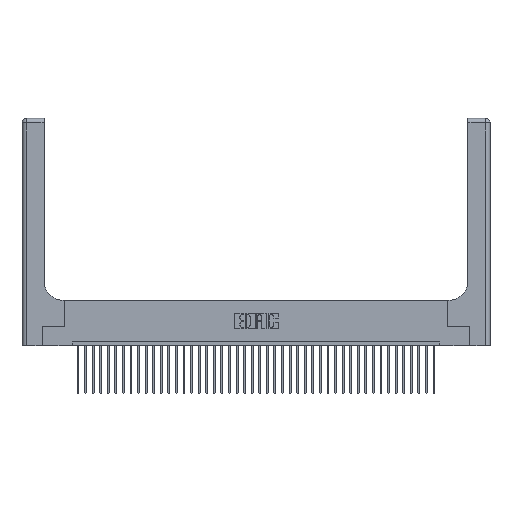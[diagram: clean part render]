
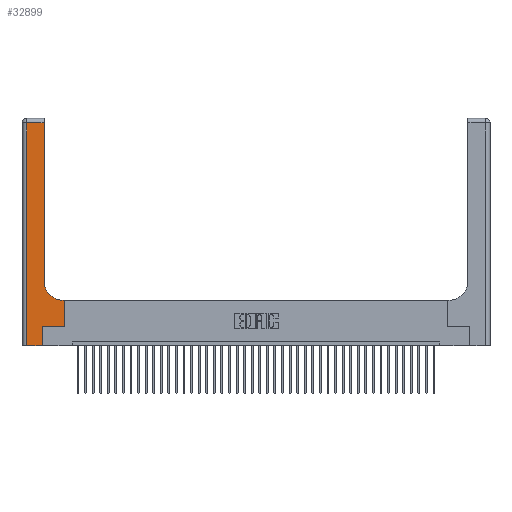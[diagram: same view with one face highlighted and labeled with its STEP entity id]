
A CAD part, top view. The second image highlights one B-rep face of the part: STEP entity #32899.
In plain terms, the highlighted planar face has unit normal (0, 0, 1).
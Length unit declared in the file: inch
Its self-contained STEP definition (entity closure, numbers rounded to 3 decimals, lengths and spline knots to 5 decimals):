
#25 = LINE ( 'NONE', #28274, #21069 ) ;
#470 = ORIENTED_EDGE ( 'NONE', *, *, #32537, .T. ) ;
#648 = CARTESIAN_POINT ( 'NONE',  ( 0., 2.94, 0.37 ) ) ;
#672 = DIRECTION ( 'NONE',  ( 0., 0., -1. ) ) ;
#700 = CARTESIAN_POINT ( 'NONE',  ( 0.269, 0.25, 0.37 ) ) ;
#2259 = CARTESIAN_POINT ( 'NONE',  ( 0.269, 0., 0.37 ) ) ;
#2383 = CARTESIAN_POINT ( 'NONE',  ( 0.5585, 0.6, 0.37 ) ) ;
#2815 = DIRECTION ( 'NONE',  ( 1., 0., 0. ) ) ;
#3543 = DIRECTION ( 'NONE',  ( 0., 1., 0. ) ) ;
#3746 = VERTEX_POINT ( 'NONE', #5873 ) ;
#4926 = LINE ( 'NONE', #5613, #18164 ) ;
#5576 = DIRECTION ( 'NONE',  ( 1., 0., 0. ) ) ;
#5613 = CARTESIAN_POINT ( 'NONE',  ( 0.06, 3., 0.37 ) ) ;
#5708 = VERTEX_POINT ( 'NONE', #24587 ) ;
#5873 = CARTESIAN_POINT ( 'NONE',  ( 0.5415, 0.6, 0.37 ) ) ;
#5874 = CARTESIAN_POINT ( 'NONE',  ( 0.06, 0., 0.37 ) ) ;
#6068 = ORIENTED_EDGE ( 'NONE', *, *, #31612, .T. ) ;
#6712 = CARTESIAN_POINT ( 'NONE',  ( 0., 3., 0.37 ) ) ;
#6886 = VECTOR ( 'NONE', #3543, 39.37008 ) ;
#9248 = LINE ( 'NONE', #35840, #23408 ) ;
#10217 = EDGE_CURVE ( 'NONE', #30166, #11776, #25, .T. ) ;
#10220 = ORIENTED_EDGE ( 'NONE', *, *, #34628, .T. ) ;
#10222 = VECTOR ( 'NONE', #38254, 39.37008 ) ;
#10480 = CARTESIAN_POINT ( 'NONE',  ( 0.06, 2.94, 0.37 ) ) ;
#10695 = EDGE_CURVE ( 'NONE', #19285, #37135, #11729, .T. ) ;
#11729 = LINE ( 'NONE', #14682, #14678 ) ;
#11776 = VERTEX_POINT ( 'NONE', #17389 ) ;
#12494 = ORIENTED_EDGE ( 'NONE', *, *, #20137, .T. ) ;
#12866 = DIRECTION ( 'NONE',  ( -1., 0., 0. ) ) ;
#13947 = DIRECTION ( 'NONE',  ( -1., 0., 0. ) ) ;
#14678 = VECTOR ( 'NONE', #36546, 39.37008 ) ;
#14682 = CARTESIAN_POINT ( 'NONE',  ( 0.5585, 0.25, 0.37 ) ) ;
#17389 = CARTESIAN_POINT ( 'NONE',  ( 0.2915, 2.94, 0.37 ) ) ;
#17453 = EDGE_LOOP ( 'NONE', ( #28823, #470, #31458, #32103, #6068, #10220, #19731, #12494, #32538 ) ) ;
#18164 = VECTOR ( 'NONE', #38486, 39.37008 ) ;
#19285 = VERTEX_POINT ( 'NONE', #28816 ) ;
#19404 = PLANE ( 'NONE',  #37772 ) ;
#19469 = EDGE_CURVE ( 'NONE', #19554, #26145, #4926, .T. ) ;
#19554 = VERTEX_POINT ( 'NONE', #10480 ) ;
#19731 = ORIENTED_EDGE ( 'NONE', *, *, #10695, .T. ) ;
#20137 = EDGE_CURVE ( 'NONE', #37135, #3746, #37638, .T. ) ;
#20225 = DIRECTION ( 'NONE',  ( 1., 0., 0. ) ) ;
#21021 = VECTOR ( 'NONE', #13947, 39.37008 ) ;
#21069 = VECTOR ( 'NONE', #28404, 39.37008 ) ;
#22883 = LINE ( 'NONE', #36173, #34190 ) ;
#23408 = VECTOR ( 'NONE', #20225, 39.37008 ) ;
#23520 = EDGE_CURVE ( 'NONE', #3746, #30166, #30486, .T. ) ;
#24570 = AXIS2_PLACEMENT_3D ( 'NONE', #37164, #27361, #5576 ) ;
#24587 = CARTESIAN_POINT ( 'NONE',  ( 0.269, 0., 0.37 ) ) ;
#25983 = CARTESIAN_POINT ( 'NONE',  ( 0.2915, 0.85, 0.37 ) ) ;
#26145 = VERTEX_POINT ( 'NONE', #5874 ) ;
#27361 = DIRECTION ( 'NONE',  ( 0., 0., -1. ) ) ;
#28274 = CARTESIAN_POINT ( 'NONE',  ( 0.2915, 3., 0.37 ) ) ;
#28404 = DIRECTION ( 'NONE',  ( 0., 1., 0. ) ) ;
#28816 = CARTESIAN_POINT ( 'NONE',  ( 0.5585, 0.25, 0.37 ) ) ;
#28823 = ORIENTED_EDGE ( 'NONE', *, *, #10217, .T. ) ;
#30166 = VERTEX_POINT ( 'NONE', #25983 ) ;
#30486 = CIRCLE ( 'NONE', #24570, 0.25 ) ;
#30837 = FACE_OUTER_BOUND ( 'NONE', #17453, .T. ) ;
#31458 = ORIENTED_EDGE ( 'NONE', *, *, #19469, .T. ) ;
#31612 = EDGE_CURVE ( 'NONE', #5708, #39168, #32355, .T. ) ;
#32103 = ORIENTED_EDGE ( 'NONE', *, *, #33302, .T. ) ;
#32355 = LINE ( 'NONE', #2259, #6886 ) ;
#32537 = EDGE_CURVE ( 'NONE', #11776, #19554, #37622, .T. ) ;
#32538 = ORIENTED_EDGE ( 'NONE', *, *, #23520, .T. ) ;
#32728 = CARTESIAN_POINT ( 'NONE',  ( 0.2915, 0.6, 0.37 ) ) ;
#32899 = ADVANCED_FACE ( 'NONE', ( #30837 ), #19404, .F. ) ;
#33302 = EDGE_CURVE ( 'NONE', #26145, #5708, #22883, .T. ) ;
#34190 = VECTOR ( 'NONE', #2815, 39.37008 ) ;
#34628 = EDGE_CURVE ( 'NONE', #39168, #19285, #9248, .T. ) ;
#35840 = CARTESIAN_POINT ( 'NONE',  ( 0.269, 0.25, 0.37 ) ) ;
#36173 = CARTESIAN_POINT ( 'NONE',  ( 0., 0., 0.37 ) ) ;
#36546 = DIRECTION ( 'NONE',  ( 0., 1., 0. ) ) ;
#37135 = VERTEX_POINT ( 'NONE', #2383 ) ;
#37164 = CARTESIAN_POINT ( 'NONE',  ( 0.5415, 0.85, 0.37 ) ) ;
#37622 = LINE ( 'NONE', #648, #10222 ) ;
#37638 = LINE ( 'NONE', #32728, #21021 ) ;
#37772 = AXIS2_PLACEMENT_3D ( 'NONE', #6712, #672, #12866 ) ;
#38254 = DIRECTION ( 'NONE',  ( -1., 0., 0. ) ) ;
#38486 = DIRECTION ( 'NONE',  ( 0., -1., 0. ) ) ;
#39168 = VERTEX_POINT ( 'NONE', #700 ) ;
